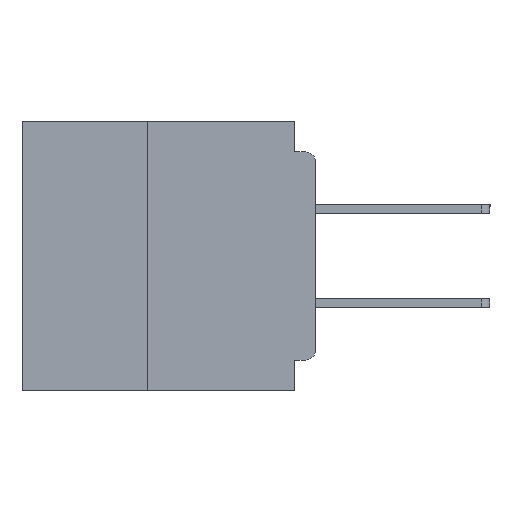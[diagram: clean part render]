
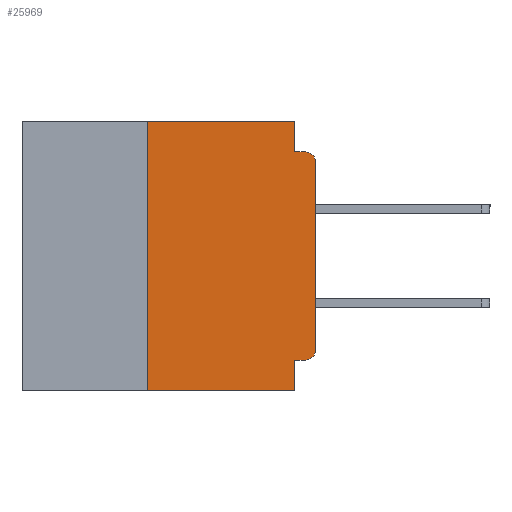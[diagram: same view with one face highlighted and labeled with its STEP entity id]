
A CAD part, left-side view. The second image highlights one B-rep face of the part: STEP entity #25969.
In plain terms, the highlighted planar face has unit normal (-1, 0, 0).
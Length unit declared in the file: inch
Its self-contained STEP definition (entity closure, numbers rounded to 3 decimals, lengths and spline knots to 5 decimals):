
#417 = VERTEX_POINT ( 'NONE', #37435 ) ;
#609 = DIRECTION ( 'NONE',  ( 0., -1., 0. ) ) ;
#675 = VERTEX_POINT ( 'NONE', #15693 ) ;
#980 = CARTESIAN_POINT ( 'NONE',  ( 0., 0.015, -0.045 ) ) ;
#997 = DIRECTION ( 'NONE',  ( 0., 0., -1. ) ) ;
#1131 = ORIENTED_EDGE ( 'NONE', *, *, #25103, .F. ) ;
#1294 = VERTEX_POINT ( 'NONE', #19300 ) ;
#1409 = ORIENTED_EDGE ( 'NONE', *, *, #2395, .F. ) ;
#1901 = AXIS2_PLACEMENT_3D ( 'NONE', #24463, #18668, #997 ) ;
#2130 = DIRECTION ( 'NONE',  ( 0., 0., 1. ) ) ;
#2198 = CARTESIAN_POINT ( 'NONE',  ( 0., 0.031, 0. ) ) ;
#2395 = EDGE_CURVE ( 'NONE', #1294, #37148, #13727, .T. ) ;
#2530 = DIRECTION ( 'NONE',  ( 0., 1., 0. ) ) ;
#2924 = CARTESIAN_POINT ( 'NONE',  ( 0., 0.031, -0.355 ) ) ;
#3317 = CARTESIAN_POINT ( 'NONE',  ( 0., 0.437, -0.4 ) ) ;
#4897 = DIRECTION ( 'NONE',  ( -1., 0., 0. ) ) ;
#5746 = CIRCLE ( 'NONE', #31664, 0.015 ) ;
#6025 = CARTESIAN_POINT ( 'NONE',  ( 0., 0., -0.045 ) ) ;
#6451 = VERTEX_POINT ( 'NONE', #6673 ) ;
#6673 = CARTESIAN_POINT ( 'NONE',  ( 0., 0.25, -0.4 ) ) ;
#6684 = CARTESIAN_POINT ( 'NONE',  ( 0., 0.015, -0.34 ) ) ;
#6766 = VECTOR ( 'NONE', #2530, 39.37008 ) ;
#6818 = CIRCLE ( 'NONE', #16521, 0.015 ) ;
#7074 = CARTESIAN_POINT ( 'NONE',  ( 0., 0.015, -0.355 ) ) ;
#7425 = LINE ( 'NONE', #2198, #36731 ) ;
#8351 = CARTESIAN_POINT ( 'NONE',  ( 0., 0.031, -0.4 ) ) ;
#9651 = DIRECTION ( 'NONE',  ( 0., 0., -1. ) ) ;
#9779 = FACE_OUTER_BOUND ( 'NONE', #10788, .T. ) ;
#9802 = VERTEX_POINT ( 'NONE', #35888 ) ;
#10727 = ORIENTED_EDGE ( 'NONE', *, *, #35765, .F. ) ;
#10788 = EDGE_LOOP ( 'NONE', ( #25252, #23556, #1409, #26361, #10727, #28717, #15937, #1131, #19187, #12722 ) ) ;
#12013 = VERTEX_POINT ( 'NONE', #22993 ) ;
#12722 = ORIENTED_EDGE ( 'NONE', *, *, #35858, .T. ) ;
#13727 = LINE ( 'NONE', #6025, #20640 ) ;
#14819 = VERTEX_POINT ( 'NONE', #37266 ) ;
#15693 = CARTESIAN_POINT ( 'NONE',  ( 0., 0.25, 0. ) ) ;
#15717 = PLANE ( 'NONE',  #1901 ) ;
#15937 = ORIENTED_EDGE ( 'NONE', *, *, #22570, .T. ) ;
#16521 = AXIS2_PLACEMENT_3D ( 'NONE', #6684, #27341, #9651 ) ;
#16869 = LINE ( 'NONE', #8351, #31438 ) ;
#17091 = LINE ( 'NONE', #3317, #31671 ) ;
#17158 = EDGE_CURVE ( 'NONE', #9802, #37148, #5746, .T. ) ;
#17338 = DIRECTION ( 'NONE',  ( 0., 0., -1. ) ) ;
#18668 = DIRECTION ( 'NONE',  ( 1., 0., 0. ) ) ;
#19187 = ORIENTED_EDGE ( 'NONE', *, *, #29758, .F. ) ;
#19300 = CARTESIAN_POINT ( 'NONE',  ( 0., 0.031, -0.045 ) ) ;
#19701 = VERTEX_POINT ( 'NONE', #2924 ) ;
#20640 = VECTOR ( 'NONE', #609, 39.37008 ) ;
#20642 = LINE ( 'NONE', #31534, #35165 ) ;
#21770 = LINE ( 'NONE', #22780, #28617 ) ;
#22570 = EDGE_CURVE ( 'NONE', #6451, #417, #17091, .T. ) ;
#22614 = CARTESIAN_POINT ( 'NONE',  ( 0., 0.015, -0.06 ) ) ;
#22780 = CARTESIAN_POINT ( 'NONE',  ( 0., 0., 0. ) ) ;
#22993 = CARTESIAN_POINT ( 'NONE',  ( 0., 0., -0.34 ) ) ;
#23556 = ORIENTED_EDGE ( 'NONE', *, *, #17158, .T. ) ;
#23981 = DIRECTION ( 'NONE',  ( 0., -1., 0. ) ) ;
#24463 = CARTESIAN_POINT ( 'NONE',  ( 0., 0.437, 0. ) ) ;
#25103 = EDGE_CURVE ( 'NONE', #19701, #417, #16869, .T. ) ;
#25252 = ORIENTED_EDGE ( 'NONE', *, *, #33748, .T. ) ;
#25578 = DIRECTION ( 'NONE',  ( 0., 0., -1. ) ) ;
#25969 = ADVANCED_FACE ( 'NONE', ( #9779 ), #15717, .F. ) ;
#26361 = ORIENTED_EDGE ( 'NONE', *, *, #27329, .F. ) ;
#27329 = EDGE_CURVE ( 'NONE', #14819, #1294, #7425, .T. ) ;
#27341 = DIRECTION ( 'NONE',  ( -1., 0., 0. ) ) ;
#28617 = VECTOR ( 'NONE', #2130, 39.37008 ) ;
#28683 = DIRECTION ( 'NONE',  ( 0., 0., -1. ) ) ;
#28717 = ORIENTED_EDGE ( 'NONE', *, *, #36791, .F. ) ;
#29758 = EDGE_CURVE ( 'NONE', #35943, #19701, #30247, .T. ) ;
#29858 = CARTESIAN_POINT ( 'NONE',  ( 0., 0.437, 0. ) ) ;
#30247 = LINE ( 'NONE', #37538, #6766 ) ;
#30680 = VECTOR ( 'NONE', #32632, 39.37008 ) ;
#31127 = LINE ( 'NONE', #29858, #30680 ) ;
#31438 = VECTOR ( 'NONE', #17338, 39.37008 ) ;
#31534 = CARTESIAN_POINT ( 'NONE',  ( 0., 0.25, -0.4 ) ) ;
#31664 = AXIS2_PLACEMENT_3D ( 'NONE', #22614, #4897, #25578 ) ;
#31671 = VECTOR ( 'NONE', #23981, 39.37008 ) ;
#32632 = DIRECTION ( 'NONE',  ( 0., -1., 0. ) ) ;
#33748 = EDGE_CURVE ( 'NONE', #12013, #9802, #21770, .T. ) ;
#34470 = DIRECTION ( 'NONE',  ( 0., 0., 1. ) ) ;
#35165 = VECTOR ( 'NONE', #34470, 39.37008 ) ;
#35765 = EDGE_CURVE ( 'NONE', #675, #14819, #31127, .T. ) ;
#35858 = EDGE_CURVE ( 'NONE', #35943, #12013, #6818, .T. ) ;
#35888 = CARTESIAN_POINT ( 'NONE',  ( 0., 0., -0.06 ) ) ;
#35943 = VERTEX_POINT ( 'NONE', #7074 ) ;
#36731 = VECTOR ( 'NONE', #28683, 39.37008 ) ;
#36791 = EDGE_CURVE ( 'NONE', #6451, #675, #20642, .T. ) ;
#37148 = VERTEX_POINT ( 'NONE', #980 ) ;
#37266 = CARTESIAN_POINT ( 'NONE',  ( 0., 0.031, 0. ) ) ;
#37435 = CARTESIAN_POINT ( 'NONE',  ( 0., 0.031, -0.4 ) ) ;
#37538 = CARTESIAN_POINT ( 'NONE',  ( 0., 0., -0.355 ) ) ;
